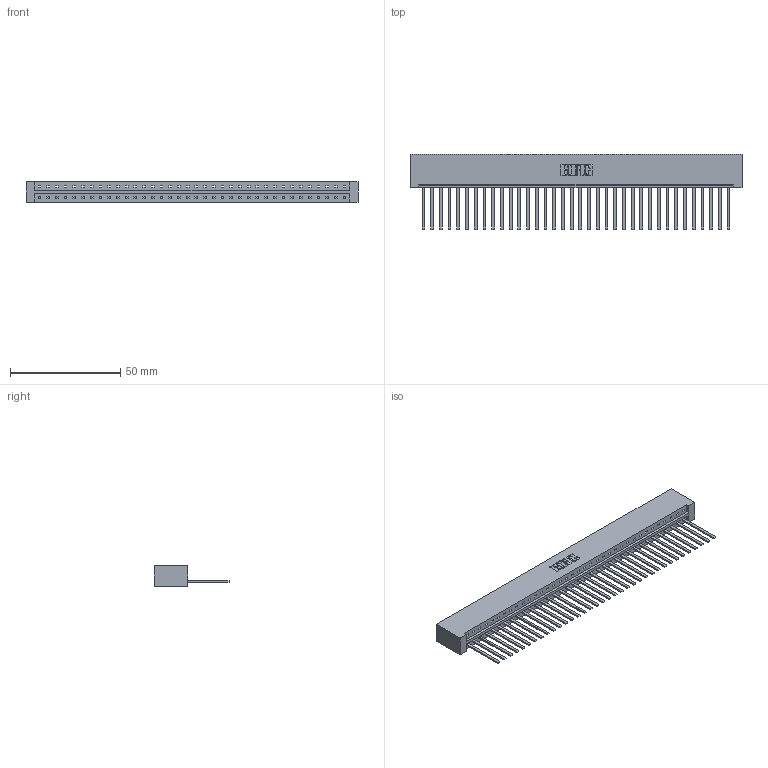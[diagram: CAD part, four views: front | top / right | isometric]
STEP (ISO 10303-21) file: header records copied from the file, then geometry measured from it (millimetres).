
FILE_DESCRIPTION (( 'STEP AP203' ), '1' );
FILE_NAME ('833-036-544-101.STEP', '2020-06-03T03:21:15', ( '' ), ( '' ), 'SwSTEP 2.0', 'SolidWorks 2020', '' );
FILE_SCHEMA (( 'CONFIG_CONTROL_DESIGN' ));
Length unit declared in the file: inch
Products named in the file (3): 345-292-001_345-293-144; 833-036-544-101; 833 Part_Lugless
Assembly tree (37 placements, depth 2):
  833-036-544-101
    833 Part_Lugless
    345-292-001_345-293-144  x36
Bounding box: 150.9 x 34.3 x 9.4 mm (x, y, z)
Volume: 16163 mm3; surface area: 18761.1 mm2
Topology: 37 solids, 37 shells, 1978 faces, 5975 edges, 3934 vertices
Faces by surface type: plane 1434, cylinder 544
Entity records: 22323 total; most frequent: CARTESIAN_POINT 3858, ORIENTED_EDGE 3830, DIRECTION 3255, EDGE_CURVE 1915, LINE 1799, VECTOR 1799, VERTEX_POINT 1274, AXIS2_PLACEMENT_3D 728
